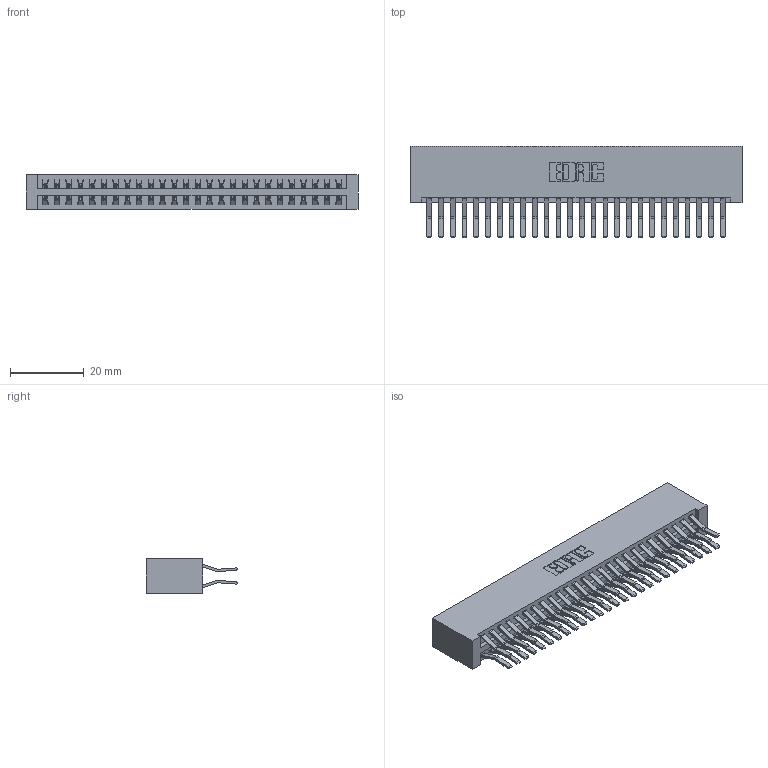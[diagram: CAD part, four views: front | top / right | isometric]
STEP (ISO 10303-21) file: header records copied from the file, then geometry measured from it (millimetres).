
FILE_DESCRIPTION (( 'STEP AP203' ), '1' );
FILE_NAME ('396-052-560-201.STEP', '2018-09-08T07:11:04', ( '' ), ( '' ), 'SwSTEP 2.0', 'SolidWorks 2016', '' );
FILE_SCHEMA (( 'CONFIG_CONTROL_DESIGN' ));
Length unit declared in the file: inch
Products named in the file (3): 396-052-560-201; 346 Part_No Mounting Lugs; 345-292-001_560 Tail
Assembly tree (53 placements, depth 2):
  396-052-560-201
    346 Part_No Mounting Lugs
    345-292-001_560 Tail  x52
Bounding box: 89.79 x 24.78 x 9.4 mm (x, y, z)
Volume: 9545.4 mm3; surface area: 13941.8 mm2
Topology: 53 solids, 53 shells, 2922 faces, 8677 edges, 5714 vertices
Faces by surface type: plane 1892, cylinder 1030
Entity records: 18933 total; most frequent: CARTESIAN_POINT 3140, ORIENTED_EDGE 3074, DIRECTION 2817, EDGE_CURVE 1537, VECTOR 1305, LINE 1305, VERTEX_POINT 1022, AXIS2_PLACEMENT_3D 756
